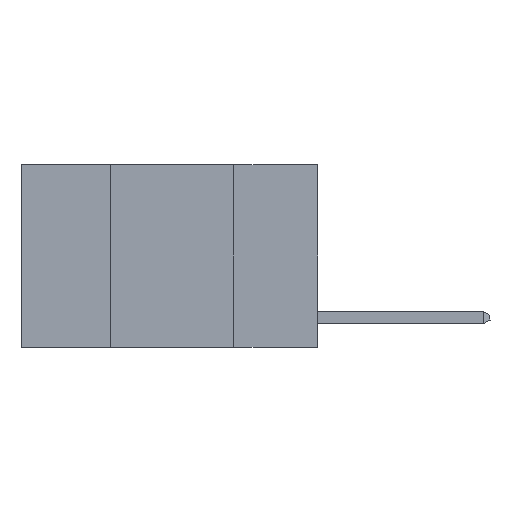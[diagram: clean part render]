
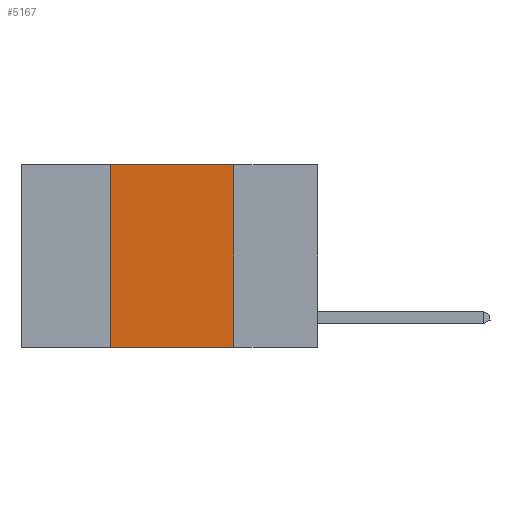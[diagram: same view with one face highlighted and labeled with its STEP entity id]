
A CAD part, left-side view. The second image highlights one B-rep face of the part: STEP entity #5167.
In plain terms, the highlighted planar face has unit normal (-1, 0, 0).
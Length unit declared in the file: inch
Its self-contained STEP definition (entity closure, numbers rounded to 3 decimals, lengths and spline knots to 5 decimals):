
#343 = CARTESIAN_POINT ( 'NONE',  ( 0., 0.17, -0.37 ) ) ;
#778 = CARTESIAN_POINT ( 'NONE',  ( 0., 0.17, 0. ) ) ;
#1643 = CARTESIAN_POINT ( 'NONE',  ( 0., 0.6, 0. ) ) ;
#2241 = CARTESIAN_POINT ( 'NONE',  ( 0., 0.6, 0. ) ) ;
#2411 = CARTESIAN_POINT ( 'NONE',  ( 0., 0.42, -0.37 ) ) ;
#2468 = DIRECTION ( 'NONE',  ( 0., 0., -1. ) ) ;
#2758 = EDGE_CURVE ( 'NONE', #12726, #11219, #15360, .T. ) ;
#4478 = VECTOR ( 'NONE', #2468, 39.37008 ) ;
#5044 = DIRECTION ( 'NONE',  ( 0., 0., -1. ) ) ;
#5167 = ADVANCED_FACE ( 'NONE', ( #10551 ), #11639, .F. ) ;
#5520 = CARTESIAN_POINT ( 'NONE',  ( 0., 0.17, 0. ) ) ;
#7153 = DIRECTION ( 'NONE',  ( 0., 0., 1. ) ) ;
#7316 = CARTESIAN_POINT ( 'NONE',  ( 0., 0.6, -0.37 ) ) ;
#9294 = CARTESIAN_POINT ( 'NONE',  ( 0., 0.42, 0. ) ) ;
#9371 = EDGE_CURVE ( 'NONE', #11219, #18647, #19963, .T. ) ;
#10097 = ORIENTED_EDGE ( 'NONE', *, *, #12644, .T. ) ;
#10420 = VERTEX_POINT ( 'NONE', #343 ) ;
#10551 = FACE_OUTER_BOUND ( 'NONE', #11165, .T. ) ;
#10569 = EDGE_CURVE ( 'NONE', #18647, #10420, #17595, .T. ) ;
#10902 = ORIENTED_EDGE ( 'NONE', *, *, #10569, .F. ) ;
#11046 = VECTOR ( 'NONE', #7153, 39.37008 ) ;
#11165 = EDGE_LOOP ( 'NONE', ( #10902, #11912, #12413, #10097 ) ) ;
#11219 = VERTEX_POINT ( 'NONE', #9294 ) ;
#11639 = PLANE ( 'NONE',  #15033 ) ;
#11912 = ORIENTED_EDGE ( 'NONE', *, *, #9371, .F. ) ;
#12413 = ORIENTED_EDGE ( 'NONE', *, *, #2758, .F. ) ;
#12644 = EDGE_CURVE ( 'NONE', #12726, #10420, #15008, .T. ) ;
#12726 = VERTEX_POINT ( 'NONE', #2411 ) ;
#13905 = DIRECTION ( 'NONE',  ( 0., -1., 0. ) ) ;
#14912 = DIRECTION ( 'NONE',  ( 1., 0., 0. ) ) ;
#15008 = LINE ( 'NONE', #7316, #18811 ) ;
#15033 = AXIS2_PLACEMENT_3D ( 'NONE', #1643, #14912, #5044 ) ;
#15286 = CARTESIAN_POINT ( 'NONE',  ( 0., 0.42, 0. ) ) ;
#15360 = LINE ( 'NONE', #15286, #11046 ) ;
#15629 = VECTOR ( 'NONE', #13905, 39.37008 ) ;
#17595 = LINE ( 'NONE', #778, #4478 ) ;
#18647 = VERTEX_POINT ( 'NONE', #5520 ) ;
#18708 = DIRECTION ( 'NONE',  ( 0., -1., 0. ) ) ;
#18811 = VECTOR ( 'NONE', #18708, 39.37008 ) ;
#19963 = LINE ( 'NONE', #2241, #15629 ) ;
